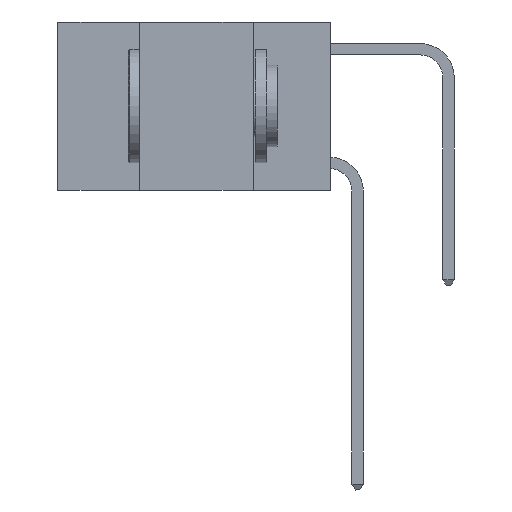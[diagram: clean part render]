
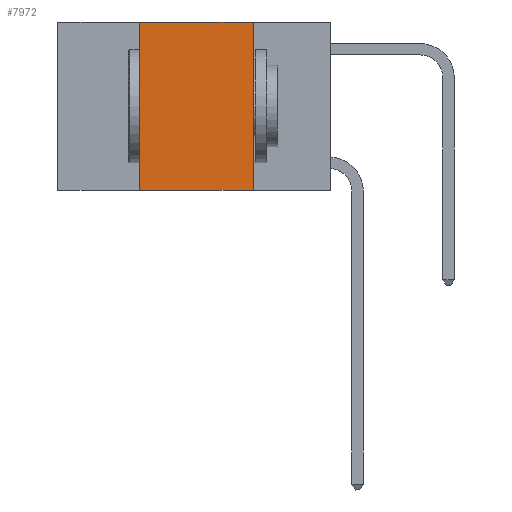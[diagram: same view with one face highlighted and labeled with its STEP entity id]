
A CAD part, left-side view. The second image highlights one B-rep face of the part: STEP entity #7972.
In plain terms, the highlighted planar face has unit normal (-1, 0, 0).
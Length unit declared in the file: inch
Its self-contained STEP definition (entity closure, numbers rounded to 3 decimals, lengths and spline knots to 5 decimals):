
#110 = ORIENTED_EDGE ( 'NONE', *, *, #471, .F. ) ;
#130 = ORIENTED_EDGE ( 'NONE', *, *, #6949, .T. ) ;
#352 = CARTESIAN_POINT ( 'NONE',  ( 0., 0.42, -0.37 ) ) ;
#414 = CARTESIAN_POINT ( 'NONE',  ( 0., 0.17, -0.37 ) ) ;
#471 = EDGE_CURVE ( 'NONE', #11815, #1450, #5332, .T. ) ;
#1203 = ORIENTED_EDGE ( 'NONE', *, *, #1958, .F. ) ;
#1450 = VERTEX_POINT ( 'NONE', #3543 ) ;
#1579 = AXIS2_PLACEMENT_3D ( 'NONE', #13187, #8974, #1797 ) ;
#1797 = DIRECTION ( 'NONE',  ( 0., 0., -1. ) ) ;
#1909 = VECTOR ( 'NONE', #9629, 39.37008 ) ;
#1927 = PLANE ( 'NONE',  #1579 ) ;
#1958 = EDGE_CURVE ( 'NONE', #1450, #9163, #7866, .T. ) ;
#2055 = VECTOR ( 'NONE', #13093, 39.37008 ) ;
#2260 = DIRECTION ( 'NONE',  ( 0., -1., 0. ) ) ;
#2374 = CARTESIAN_POINT ( 'NONE',  ( 0., 0.42, 0. ) ) ;
#3543 = CARTESIAN_POINT ( 'NONE',  ( 0., 0.42, 0. ) ) ;
#4955 = VECTOR ( 'NONE', #6068, 39.37008 ) ;
#5332 = LINE ( 'NONE', #2374, #1909 ) ;
#6026 = FACE_OUTER_BOUND ( 'NONE', #8472, .T. ) ;
#6068 = DIRECTION ( 'NONE',  ( 0., 0., -1. ) ) ;
#6508 = CARTESIAN_POINT ( 'NONE',  ( 0., 0.17, 0. ) ) ;
#6949 = EDGE_CURVE ( 'NONE', #11815, #11780, #12499, .T. ) ;
#6963 = VECTOR ( 'NONE', #2260, 39.37008 ) ;
#7355 = CARTESIAN_POINT ( 'NONE',  ( 0., 0.6, -0.37 ) ) ;
#7866 = LINE ( 'NONE', #9896, #2055 ) ;
#7972 = ADVANCED_FACE ( 'NONE', ( #6026 ), #1927, .F. ) ;
#8472 = EDGE_LOOP ( 'NONE', ( #12263, #1203, #110, #130 ) ) ;
#8974 = DIRECTION ( 'NONE',  ( 1., 0., 0. ) ) ;
#9163 = VERTEX_POINT ( 'NONE', #6508 ) ;
#9629 = DIRECTION ( 'NONE',  ( 0., 0., 1. ) ) ;
#9896 = CARTESIAN_POINT ( 'NONE',  ( 0., 0.6, 0. ) ) ;
#11234 = CARTESIAN_POINT ( 'NONE',  ( 0., 0.17, 0. ) ) ;
#11780 = VERTEX_POINT ( 'NONE', #414 ) ;
#11815 = VERTEX_POINT ( 'NONE', #352 ) ;
#12232 = LINE ( 'NONE', #11234, #4955 ) ;
#12263 = ORIENTED_EDGE ( 'NONE', *, *, #12610, .F. ) ;
#12499 = LINE ( 'NONE', #7355, #6963 ) ;
#12610 = EDGE_CURVE ( 'NONE', #9163, #11780, #12232, .T. ) ;
#13093 = DIRECTION ( 'NONE',  ( 0., -1., 0. ) ) ;
#13187 = CARTESIAN_POINT ( 'NONE',  ( 0., 0.6, 0. ) ) ;
